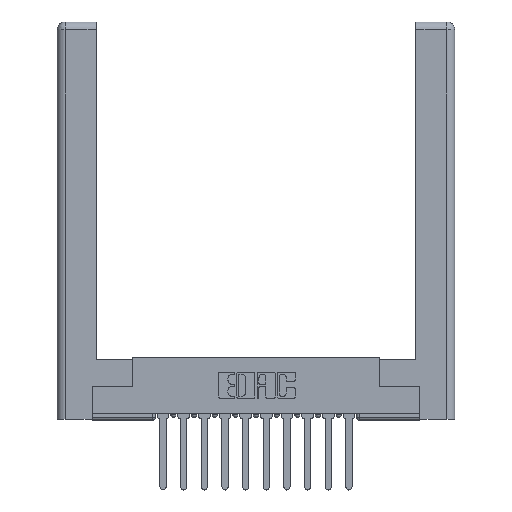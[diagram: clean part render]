
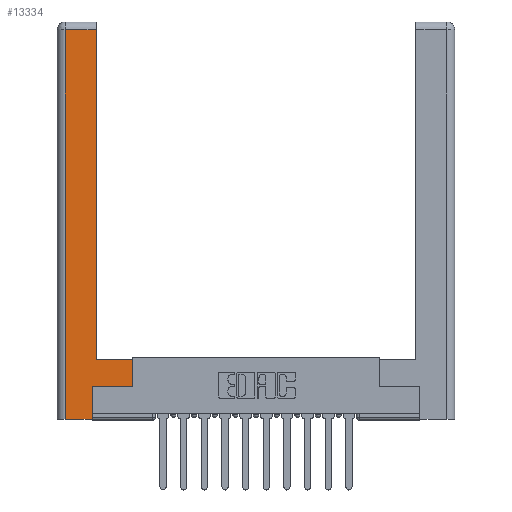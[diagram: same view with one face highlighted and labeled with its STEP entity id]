
A CAD part, top view. The second image highlights one B-rep face of the part: STEP entity #13334.
In plain terms, the highlighted planar face has unit normal (0, 0, 1).
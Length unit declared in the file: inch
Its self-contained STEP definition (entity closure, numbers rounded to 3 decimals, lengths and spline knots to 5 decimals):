
#157 = LINE ( 'NONE', #9190, #9260 ) ;
#188 = VECTOR ( 'NONE', #10305, 39.37008 ) ;
#334 = VECTOR ( 'NONE', #3774, 39.37008 ) ;
#500 = EDGE_CURVE ( 'NONE', #4308, #8491, #8157, .T. ) ;
#624 = VERTEX_POINT ( 'NONE', #2950 ) ;
#642 = CARTESIAN_POINT ( 'NONE',  ( 0.0615, 2.94, 0. ) ) ;
#709 = LINE ( 'NONE', #1312, #334 ) ;
#837 = DIRECTION ( 'NONE',  ( -1., 0., 0. ) ) ;
#1312 = CARTESIAN_POINT ( 'NONE',  ( 0.265, 0., 0. ) ) ;
#1599 = CARTESIAN_POINT ( 'NONE',  ( 0.265, 0.245, 0. ) ) ;
#1732 = CARTESIAN_POINT ( 'NONE',  ( 0.565, 0.45, 0. ) ) ;
#1765 = ORIENTED_EDGE ( 'NONE', *, *, #500, .T. ) ;
#2250 = LINE ( 'NONE', #8292, #7840 ) ;
#2543 = VERTEX_POINT ( 'NONE', #1599 ) ;
#2950 = CARTESIAN_POINT ( 'NONE',  ( 0.265, 0., 0. ) ) ;
#2977 = VERTEX_POINT ( 'NONE', #10959 ) ;
#3339 = VERTEX_POINT ( 'NONE', #8218 ) ;
#3384 = ORIENTED_EDGE ( 'NONE', *, *, #10202, .T. ) ;
#3391 = DIRECTION ( 'NONE',  ( 0., -1., 0. ) ) ;
#3584 = DIRECTION ( 'NONE',  ( 0., 1., 0. ) ) ;
#3688 = CARTESIAN_POINT ( 'NONE',  ( 0.295, 3., 0. ) ) ;
#3708 = LINE ( 'NONE', #15162, #15280 ) ;
#3774 = DIRECTION ( 'NONE',  ( 1., 0., 0. ) ) ;
#4166 = AXIS2_PLACEMENT_3D ( 'NONE', #4522, #9370, #5864 ) ;
#4308 = VERTEX_POINT ( 'NONE', #10499 ) ;
#4522 = CARTESIAN_POINT ( 'NONE',  ( 0., 0., 0. ) ) ;
#4655 = FACE_OUTER_BOUND ( 'NONE', #7596, .T. ) ;
#4971 = VECTOR ( 'NONE', #5187, 39.37008 ) ;
#5187 = DIRECTION ( 'NONE',  ( 0., 1., 0. ) ) ;
#5704 = PLANE ( 'NONE',  #4166 ) ;
#5864 = DIRECTION ( 'NONE',  ( -1., 0., 0. ) ) ;
#6466 = ORIENTED_EDGE ( 'NONE', *, *, #10275, .T. ) ;
#6608 = ORIENTED_EDGE ( 'NONE', *, *, #11142, .T. ) ;
#6869 = LINE ( 'NONE', #3688, #9685 ) ;
#7442 = LINE ( 'NONE', #15000, #188 ) ;
#7596 = EDGE_LOOP ( 'NONE', ( #11894, #10098, #14554, #6608, #14704, #6466, #1765, #3384 ) ) ;
#7715 = CARTESIAN_POINT ( 'NONE',  ( 0.295, 0.45, 0. ) ) ;
#7840 = VECTOR ( 'NONE', #3391, 39.37008 ) ;
#8157 = LINE ( 'NONE', #1732, #4971 ) ;
#8218 = CARTESIAN_POINT ( 'NONE',  ( 0.0615, 0., 0. ) ) ;
#8242 = EDGE_CURVE ( 'NONE', #13022, #2977, #6869, .T. ) ;
#8292 = CARTESIAN_POINT ( 'NONE',  ( 0.0615, 0., 0. ) ) ;
#8491 = VERTEX_POINT ( 'NONE', #13257 ) ;
#9094 = LINE ( 'NONE', #7715, #10610 ) ;
#9190 = CARTESIAN_POINT ( 'NONE',  ( 0.265, 0.245, 0. ) ) ;
#9260 = VECTOR ( 'NONE', #12585, 39.37008 ) ;
#9335 = VERTEX_POINT ( 'NONE', #642 ) ;
#9370 = DIRECTION ( 'NONE',  ( 0., 0., -1. ) ) ;
#9398 = EDGE_CURVE ( 'NONE', #624, #2543, #157, .T. ) ;
#9485 = EDGE_CURVE ( 'NONE', #2977, #9335, #3708, .T. ) ;
#9685 = VECTOR ( 'NONE', #3584, 39.37008 ) ;
#10098 = ORIENTED_EDGE ( 'NONE', *, *, #9485, .T. ) ;
#10202 = EDGE_CURVE ( 'NONE', #8491, #13022, #9094, .T. ) ;
#10275 = EDGE_CURVE ( 'NONE', #2543, #4308, #7442, .T. ) ;
#10305 = DIRECTION ( 'NONE',  ( 1., 0., 0. ) ) ;
#10499 = CARTESIAN_POINT ( 'NONE',  ( 0.565, 0.245, 0. ) ) ;
#10610 = VECTOR ( 'NONE', #13747, 39.37008 ) ;
#10959 = CARTESIAN_POINT ( 'NONE',  ( 0.295, 2.94, 0. ) ) ;
#11142 = EDGE_CURVE ( 'NONE', #3339, #624, #709, .T. ) ;
#11894 = ORIENTED_EDGE ( 'NONE', *, *, #8242, .T. ) ;
#12585 = DIRECTION ( 'NONE',  ( 0., 1., 0. ) ) ;
#13022 = VERTEX_POINT ( 'NONE', #13711 ) ;
#13257 = CARTESIAN_POINT ( 'NONE',  ( 0.565, 0.45, 0. ) ) ;
#13318 = EDGE_CURVE ( 'NONE', #9335, #3339, #2250, .T. ) ;
#13334 = ADVANCED_FACE ( 'NONE', ( #4655 ), #5704, .F. ) ;
#13711 = CARTESIAN_POINT ( 'NONE',  ( 0.295, 0.45, 0. ) ) ;
#13747 = DIRECTION ( 'NONE',  ( -1., 0., 0. ) ) ;
#14554 = ORIENTED_EDGE ( 'NONE', *, *, #13318, .T. ) ;
#14704 = ORIENTED_EDGE ( 'NONE', *, *, #9398, .T. ) ;
#15000 = CARTESIAN_POINT ( 'NONE',  ( 0.565, 0.245, 0. ) ) ;
#15162 = CARTESIAN_POINT ( 'NONE',  ( 0.0615, 2.94, 0. ) ) ;
#15280 = VECTOR ( 'NONE', #837, 39.37008 ) ;
